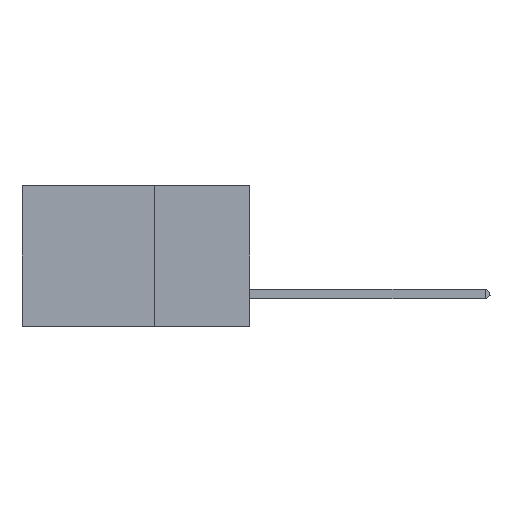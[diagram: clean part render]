
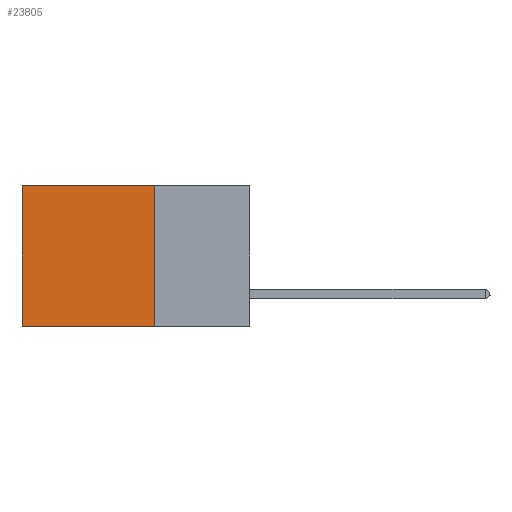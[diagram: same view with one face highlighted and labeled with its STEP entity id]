
A CAD part, left-side view. The second image highlights one B-rep face of the part: STEP entity #23805.
In plain terms, the highlighted planar face has unit normal (-1, 0, 0).
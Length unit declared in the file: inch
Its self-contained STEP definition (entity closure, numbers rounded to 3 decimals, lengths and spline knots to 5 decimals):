
#490 = DIRECTION ( 'NONE',  ( 0., 0., -1. ) ) ;
#5214 = VECTOR ( 'NONE', #33750, 39.37008 ) ;
#6903 = LINE ( 'NONE', #26863, #5214 ) ;
#9684 = EDGE_CURVE ( 'NONE', #29920, #39447, #6903, .T. ) ;
#9954 = CARTESIAN_POINT ( 'NONE',  ( 0.2875, 0.25, 0. ) ) ;
#11707 = DIRECTION ( 'NONE',  ( 1., 0., 0. ) ) ;
#11899 = ORIENTED_EDGE ( 'NONE', *, *, #9684, .F. ) ;
#12297 = ORIENTED_EDGE ( 'NONE', *, *, #33921, .T. ) ;
#12423 = CARTESIAN_POINT ( 'NONE',  ( 0.2875, 0.25, -0.37 ) ) ;
#12522 = VERTEX_POINT ( 'NONE', #38076 ) ;
#15506 = DIRECTION ( 'NONE',  ( 0., 1., 0. ) ) ;
#15921 = PLANE ( 'NONE',  #32201 ) ;
#17438 = LINE ( 'NONE', #37868, #46077 ) ;
#21274 = DIRECTION ( 'NONE',  ( 0., 1., 0. ) ) ;
#21528 = EDGE_LOOP ( 'NONE', ( #12297, #45100, #11899, #32687 ) ) ;
#23320 = CARTESIAN_POINT ( 'NONE',  ( 0.2875, 0.6, -0.37 ) ) ;
#23805 = ADVANCED_FACE ( 'NONE', ( #36200 ), #15921, .F. ) ;
#24943 = EDGE_CURVE ( 'NONE', #39447, #48004, #17438, .T. ) ;
#26396 = LINE ( 'NONE', #32305, #29277 ) ;
#26863 = CARTESIAN_POINT ( 'NONE',  ( 0.2875, 0.25, 0. ) ) ;
#28944 = CARTESIAN_POINT ( 'NONE',  ( 0.2875, 0.25, 0. ) ) ;
#29277 = VECTOR ( 'NONE', #36245, 39.37008 ) ;
#29758 = EDGE_CURVE ( 'NONE', #29920, #12522, #46271, .T. ) ;
#29920 = VERTEX_POINT ( 'NONE', #28944 ) ;
#30764 = CARTESIAN_POINT ( 'NONE',  ( 0.2875, 0.25, 0. ) ) ;
#32201 = AXIS2_PLACEMENT_3D ( 'NONE', #30764, #11707, #490 ) ;
#32305 = CARTESIAN_POINT ( 'NONE',  ( 0.2875, 0.6, 0. ) ) ;
#32687 = ORIENTED_EDGE ( 'NONE', *, *, #29758, .T. ) ;
#33750 = DIRECTION ( 'NONE',  ( 0., 0., -1. ) ) ;
#33921 = EDGE_CURVE ( 'NONE', #12522, #48004, #26396, .T. ) ;
#36200 = FACE_OUTER_BOUND ( 'NONE', #21528, .T. ) ;
#36245 = DIRECTION ( 'NONE',  ( 0., 0., -1. ) ) ;
#37868 = CARTESIAN_POINT ( 'NONE',  ( 0.2875, 0.25, -0.37 ) ) ;
#38076 = CARTESIAN_POINT ( 'NONE',  ( 0.2875, 0.6, 0. ) ) ;
#39447 = VERTEX_POINT ( 'NONE', #12423 ) ;
#42744 = VECTOR ( 'NONE', #21274, 39.37008 ) ;
#45100 = ORIENTED_EDGE ( 'NONE', *, *, #24943, .F. ) ;
#46077 = VECTOR ( 'NONE', #15506, 39.37008 ) ;
#46271 = LINE ( 'NONE', #9954, #42744 ) ;
#48004 = VERTEX_POINT ( 'NONE', #23320 ) ;
